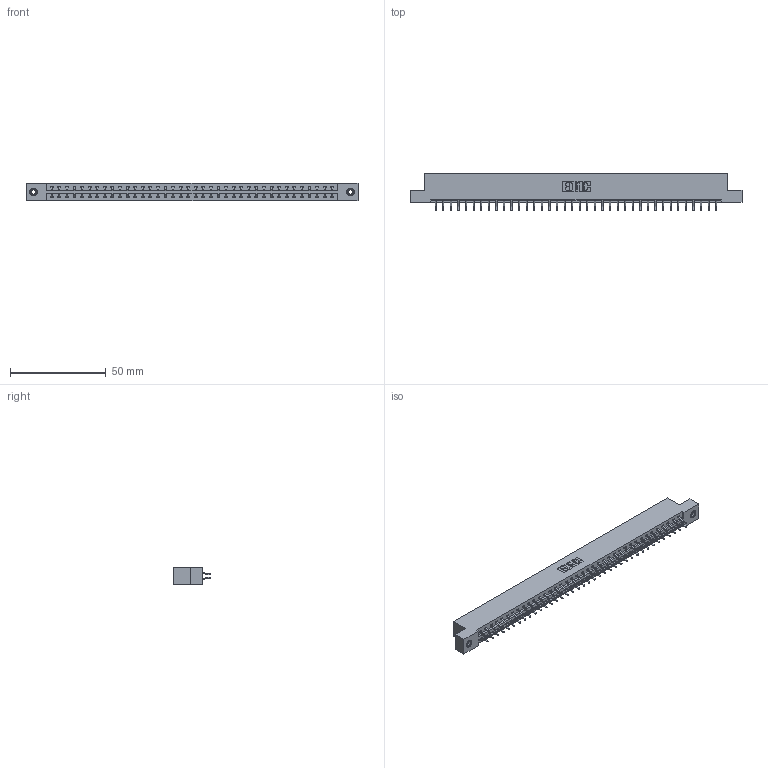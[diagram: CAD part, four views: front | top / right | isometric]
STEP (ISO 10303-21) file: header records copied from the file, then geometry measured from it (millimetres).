
FILE_DESCRIPTION (( 'STEP AP203' ), '1' );
FILE_NAME ('337-076-556-208.STEP', '2019-10-10T10:54:03', ( '' ), ( '' ), 'SwSTEP 2.0', 'SolidWorks 2016', '' );
FILE_SCHEMA (( 'CONFIG_CONTROL_DESIGN' ));
Length unit declared in the file: inch
Products named in the file (4): 345-250-001_345-250-003-102; 337-076-556-208; 345-292-001_556 Tail; 337 Part_Flush Mounting Lugs - 0.156 Dia-TI
Assembly tree (79 placements, depth 2):
  337-076-556-208
    337 Part_Flush Mounting Lugs - 0.156 Dia-TI
    345-292-001_556 Tail  x76
    345-250-001_345-250-003-102  x2
Bounding box: 173.58 x 19.57 x 9.4 mm (x, y, z)
Volume: 18230.8 mm3; surface area: 20514.9 mm2
Topology: 79 solids, 79 shells, 4734 faces, 14051 edges, 9258 vertices
Faces by surface type: plane 3294, cylinder 1424, cone 12, torus 4
Entity records: 31386 total; most frequent: CARTESIAN_POINT 5285, ORIENTED_EDGE 5202, DIRECTION 4523, EDGE_CURVE 2601, VECTOR 2445, LINE 2445, VERTEX_POINT 1728, AXIS2_PLACEMENT_3D 1039
